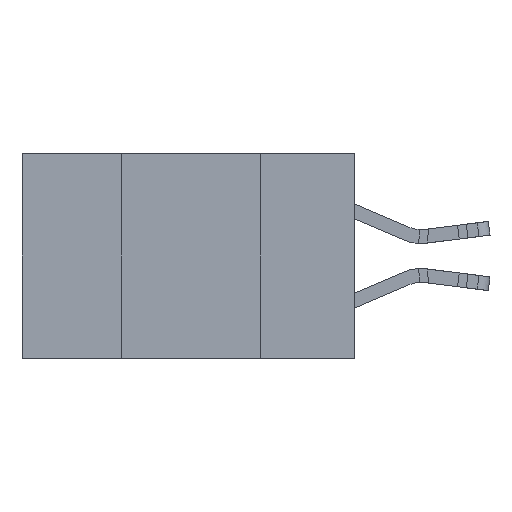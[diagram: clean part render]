
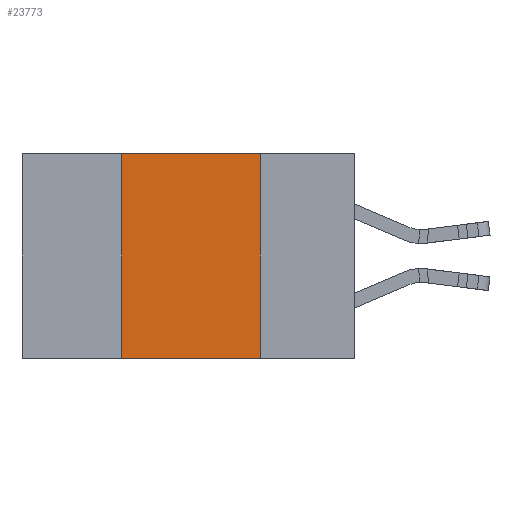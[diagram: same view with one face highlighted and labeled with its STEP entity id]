
A CAD part, left-side view. The second image highlights one B-rep face of the part: STEP entity #23773.
In plain terms, the highlighted planar face has unit normal (-1, 0, 0).
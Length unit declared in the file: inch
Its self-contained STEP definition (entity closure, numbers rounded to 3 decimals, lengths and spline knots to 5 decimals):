
#87 = VERTEX_POINT ( 'NONE', #1221 ) ;
#1221 = CARTESIAN_POINT ( 'NONE',  ( 0., 0.17, 0. ) ) ;
#1657 = CARTESIAN_POINT ( 'NONE',  ( 0., 0.17, -0.37 ) ) ;
#2019 = EDGE_CURVE ( 'NONE', #27290, #20280, #23311, .T. ) ;
#4628 = LINE ( 'NONE', #27900, #27671 ) ;
#4845 = ORIENTED_EDGE ( 'NONE', *, *, #2019, .T. ) ;
#6644 = VECTOR ( 'NONE', #10783, 39.37008 ) ;
#6925 = ORIENTED_EDGE ( 'NONE', *, *, #7873, .F. ) ;
#7873 = EDGE_CURVE ( 'NONE', #22726, #87, #4628, .T. ) ;
#10783 = DIRECTION ( 'NONE',  ( 0., 0., -1. ) ) ;
#11221 = LINE ( 'NONE', #12318, #21329 ) ;
#12136 = PLANE ( 'NONE',  #27361 ) ;
#12318 = CARTESIAN_POINT ( 'NONE',  ( 0., 0.42, 0. ) ) ;
#12415 = DIRECTION ( 'NONE',  ( 0., 0., 1. ) ) ;
#13933 = VECTOR ( 'NONE', #20433, 39.37008 ) ;
#16115 = FACE_OUTER_BOUND ( 'NONE', #24653, .T. ) ;
#16210 = DIRECTION ( 'NONE',  ( 0., -1., 0. ) ) ;
#17637 = CARTESIAN_POINT ( 'NONE',  ( 0., 0.17, 0. ) ) ;
#17880 = CARTESIAN_POINT ( 'NONE',  ( 0., 0.42, 0. ) ) ;
#18984 = ORIENTED_EDGE ( 'NONE', *, *, #27233, .F. ) ;
#19314 = CARTESIAN_POINT ( 'NONE',  ( 0., 0.6, 0. ) ) ;
#19603 = LINE ( 'NONE', #17637, #6644 ) ;
#20280 = VERTEX_POINT ( 'NONE', #1657 ) ;
#20433 = DIRECTION ( 'NONE',  ( 0., -1., 0. ) ) ;
#20673 = EDGE_CURVE ( 'NONE', #87, #20280, #19603, .T. ) ;
#21329 = VECTOR ( 'NONE', #12415, 39.37008 ) ;
#21330 = DIRECTION ( 'NONE',  ( 1., 0., 0. ) ) ;
#22289 = CARTESIAN_POINT ( 'NONE',  ( 0., 0.42, -0.37 ) ) ;
#22726 = VERTEX_POINT ( 'NONE', #17880 ) ;
#23311 = LINE ( 'NONE', #27358, #13933 ) ;
#23625 = DIRECTION ( 'NONE',  ( 0., 0., -1. ) ) ;
#23773 = ADVANCED_FACE ( 'NONE', ( #16115 ), #12136, .F. ) ;
#24653 = EDGE_LOOP ( 'NONE', ( #24904, #6925, #18984, #4845 ) ) ;
#24904 = ORIENTED_EDGE ( 'NONE', *, *, #20673, .F. ) ;
#27233 = EDGE_CURVE ( 'NONE', #27290, #22726, #11221, .T. ) ;
#27290 = VERTEX_POINT ( 'NONE', #22289 ) ;
#27358 = CARTESIAN_POINT ( 'NONE',  ( 0., 0.6, -0.37 ) ) ;
#27361 = AXIS2_PLACEMENT_3D ( 'NONE', #19314, #21330, #23625 ) ;
#27671 = VECTOR ( 'NONE', #16210, 39.37008 ) ;
#27900 = CARTESIAN_POINT ( 'NONE',  ( 0., 0.6, 0. ) ) ;
